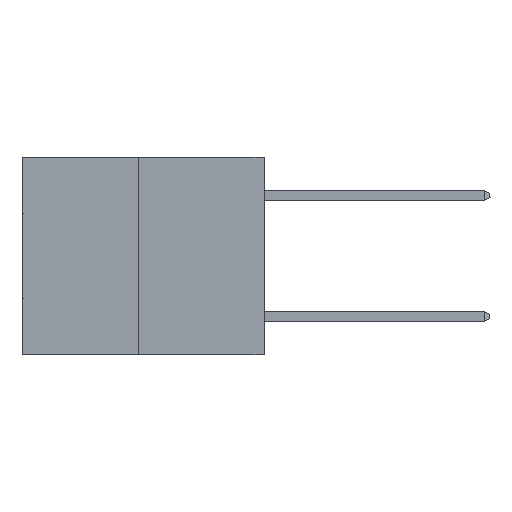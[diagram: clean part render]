
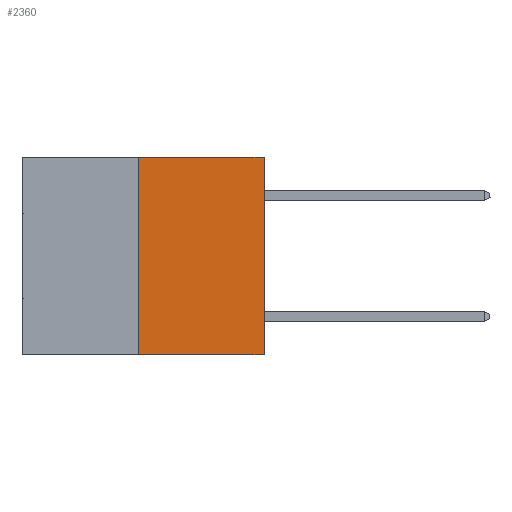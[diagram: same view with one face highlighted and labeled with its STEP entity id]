
A CAD part, left-side view. The second image highlights one B-rep face of the part: STEP entity #2360.
In plain terms, the highlighted planar face has unit normal (-1, 0, 0).
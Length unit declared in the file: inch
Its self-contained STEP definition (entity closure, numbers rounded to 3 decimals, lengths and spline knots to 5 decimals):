
#2114 = VECTOR ( 'NONE', #5121, 39.37008 ) ;
#2151 = VECTOR ( 'NONE', #23387, 39.37008 ) ;
#2360 = ADVANCED_FACE ( 'NONE', ( #7528 ), #10287, .F. ) ;
#2693 = CARTESIAN_POINT ( 'NONE',  ( 0., 0.6, 0. ) ) ;
#3398 = EDGE_CURVE ( 'NONE', #31956, #26471, #6638, .T. ) ;
#5121 = DIRECTION ( 'NONE',  ( 0., -1., 0. ) ) ;
#5239 = ORIENTED_EDGE ( 'NONE', *, *, #3398, .T. ) ;
#5639 = CARTESIAN_POINT ( 'NONE',  ( 0., 0., 0. ) ) ;
#6638 = LINE ( 'NONE', #23327, #2114 ) ;
#6936 = EDGE_LOOP ( 'NONE', ( #13280, #5239, #19355, #9048 ) ) ;
#6990 = VECTOR ( 'NONE', #32591, 39.37008 ) ;
#7388 = CARTESIAN_POINT ( 'NONE',  ( 0., 0.6, 0. ) ) ;
#7528 = FACE_OUTER_BOUND ( 'NONE', #6936, .T. ) ;
#7571 = CARTESIAN_POINT ( 'NONE',  ( 0., 0.312, 0. ) ) ;
#7613 = CARTESIAN_POINT ( 'NONE',  ( 0., 0.312, -0.49 ) ) ;
#9048 = ORIENTED_EDGE ( 'NONE', *, *, #34229, .F. ) ;
#9272 = VERTEX_POINT ( 'NONE', #7571 ) ;
#10287 = PLANE ( 'NONE',  #34317 ) ;
#10481 = VECTOR ( 'NONE', #29405, 39.37008 ) ;
#10741 = LINE ( 'NONE', #21936, #6990 ) ;
#12208 = EDGE_CURVE ( 'NONE', #26471, #19823, #10741, .T. ) ;
#13004 = DIRECTION ( 'NONE',  ( 0., 0., -1. ) ) ;
#13280 = ORIENTED_EDGE ( 'NONE', *, *, #16217, .F. ) ;
#15646 = DIRECTION ( 'NONE',  ( 1., 0., 0. ) ) ;
#15659 = CARTESIAN_POINT ( 'NONE',  ( 0., 0., -0.49 ) ) ;
#16217 = EDGE_CURVE ( 'NONE', #31956, #9272, #22554, .T. ) ;
#17433 = CARTESIAN_POINT ( 'NONE',  ( 0., 0.312, -0.49 ) ) ;
#17614 = LINE ( 'NONE', #2693, #10481 ) ;
#19355 = ORIENTED_EDGE ( 'NONE', *, *, #12208, .T. ) ;
#19823 = VERTEX_POINT ( 'NONE', #5639 ) ;
#21936 = CARTESIAN_POINT ( 'NONE',  ( 0., 0., 0. ) ) ;
#22554 = LINE ( 'NONE', #7613, #2151 ) ;
#23327 = CARTESIAN_POINT ( 'NONE',  ( 0., 0.6, -0.49 ) ) ;
#23387 = DIRECTION ( 'NONE',  ( 0., 0., 1. ) ) ;
#26471 = VERTEX_POINT ( 'NONE', #15659 ) ;
#29405 = DIRECTION ( 'NONE',  ( 0., -1., 0. ) ) ;
#31956 = VERTEX_POINT ( 'NONE', #17433 ) ;
#32591 = DIRECTION ( 'NONE',  ( 0., 0., 1. ) ) ;
#34229 = EDGE_CURVE ( 'NONE', #9272, #19823, #17614, .T. ) ;
#34317 = AXIS2_PLACEMENT_3D ( 'NONE', #7388, #15646, #13004 ) ;
